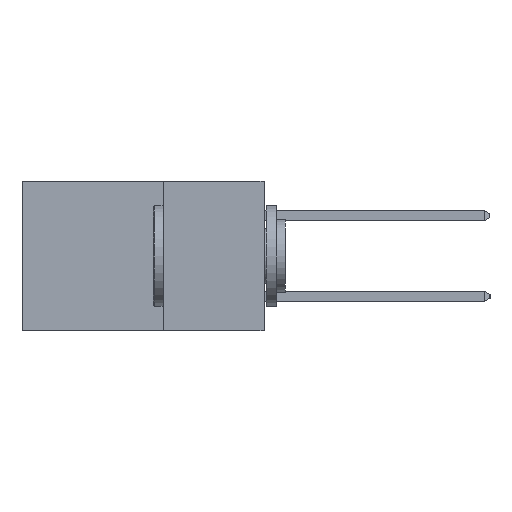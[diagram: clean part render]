
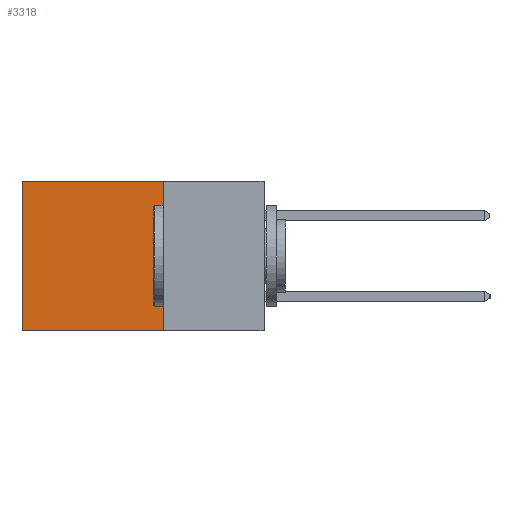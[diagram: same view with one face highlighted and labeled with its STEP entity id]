
A CAD part, left-side view. The second image highlights one B-rep face of the part: STEP entity #3318.
In plain terms, the highlighted planar face has unit normal (-1, 0, 0).
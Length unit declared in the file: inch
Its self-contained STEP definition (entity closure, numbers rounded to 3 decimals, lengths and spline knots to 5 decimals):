
#300 = EDGE_CURVE ( 'NONE', #4374, #13190, #9897, .T. ) ;
#1088 = CARTESIAN_POINT ( 'NONE',  ( 0.2615, 0.25, -0.37 ) ) ;
#1111 = DIRECTION ( 'NONE',  ( 0., 0., -1. ) ) ;
#1829 = CARTESIAN_POINT ( 'NONE',  ( 0.2615, 0.6, 0. ) ) ;
#2271 = LINE ( 'NONE', #9546, #12321 ) ;
#2806 = EDGE_CURVE ( 'NONE', #10198, #4374, #2271, .T. ) ;
#3191 = DIRECTION ( 'NONE',  ( 0., 1., 0. ) ) ;
#3207 = CARTESIAN_POINT ( 'NONE',  ( 0.2615, 0.25, -0.37 ) ) ;
#3282 = ORIENTED_EDGE ( 'NONE', *, *, #2806, .T. ) ;
#3318 = ADVANCED_FACE ( 'NONE', ( #5148 ), #12462, .F. ) ;
#3947 = CARTESIAN_POINT ( 'NONE',  ( 0.2615, 0.25, 0. ) ) ;
#4374 = VERTEX_POINT ( 'NONE', #1829 ) ;
#5003 = LINE ( 'NONE', #1088, #15076 ) ;
#5148 = FACE_OUTER_BOUND ( 'NONE', #8443, .T. ) ;
#5961 = AXIS2_PLACEMENT_3D ( 'NONE', #10969, #10917, #10878 ) ;
#6017 = DIRECTION ( 'NONE',  ( 0., 0., -1. ) ) ;
#6426 = VERTEX_POINT ( 'NONE', #8828 ) ;
#6914 = CARTESIAN_POINT ( 'NONE',  ( 0.2615, 0.6, -0.37 ) ) ;
#6985 = ORIENTED_EDGE ( 'NONE', *, *, #300, .T. ) ;
#7278 = EDGE_CURVE ( 'NONE', #6426, #13190, #13007, .T. ) ;
#7685 = DIRECTION ( 'NONE',  ( 0., 1., 0. ) ) ;
#7839 = ORIENTED_EDGE ( 'NONE', *, *, #12298, .F. ) ;
#8443 = EDGE_LOOP ( 'NONE', ( #6985, #13273, #7839, #3282 ) ) ;
#8541 = CARTESIAN_POINT ( 'NONE',  ( 0.2615, 0.6, -0.37 ) ) ;
#8828 = CARTESIAN_POINT ( 'NONE',  ( 0.2615, 0.25, -0.37 ) ) ;
#9546 = CARTESIAN_POINT ( 'NONE',  ( 0.2615, 0.25, 0. ) ) ;
#9623 = VECTOR ( 'NONE', #3191, 39.37008 ) ;
#9897 = LINE ( 'NONE', #8541, #12547 ) ;
#10198 = VERTEX_POINT ( 'NONE', #3947 ) ;
#10878 = DIRECTION ( 'NONE',  ( 0., 0., -1. ) ) ;
#10917 = DIRECTION ( 'NONE',  ( 1., 0., 0. ) ) ;
#10969 = CARTESIAN_POINT ( 'NONE',  ( 0.2615, 0.25, -0.37 ) ) ;
#12298 = EDGE_CURVE ( 'NONE', #10198, #6426, #5003, .T. ) ;
#12321 = VECTOR ( 'NONE', #7685, 39.37008 ) ;
#12462 = PLANE ( 'NONE',  #5961 ) ;
#12547 = VECTOR ( 'NONE', #6017, 39.37008 ) ;
#13007 = LINE ( 'NONE', #3207, #9623 ) ;
#13190 = VERTEX_POINT ( 'NONE', #6914 ) ;
#13273 = ORIENTED_EDGE ( 'NONE', *, *, #7278, .F. ) ;
#15076 = VECTOR ( 'NONE', #1111, 39.37008 ) ;
